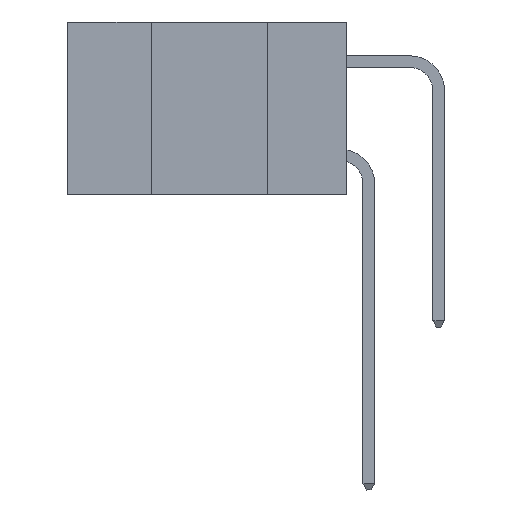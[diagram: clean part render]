
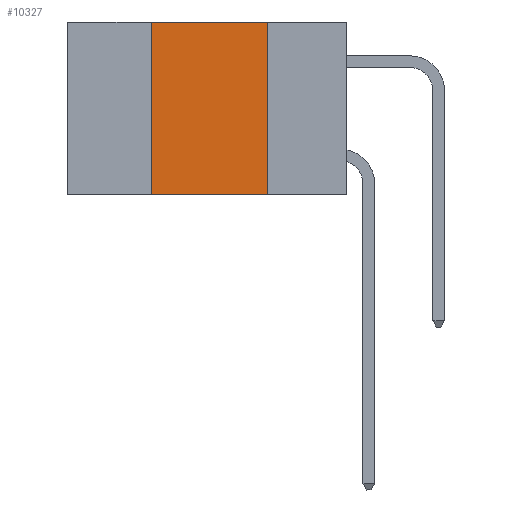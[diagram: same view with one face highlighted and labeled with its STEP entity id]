
A CAD part, left-side view. The second image highlights one B-rep face of the part: STEP entity #10327.
In plain terms, the highlighted planar face has unit normal (-1, 0, 0).
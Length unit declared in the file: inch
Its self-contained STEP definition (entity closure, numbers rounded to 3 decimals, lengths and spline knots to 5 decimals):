
#1672 = CARTESIAN_POINT ( 'NONE',  ( 0., 0.42, -0.37 ) ) ;
#1810 = CARTESIAN_POINT ( 'NONE',  ( 0., 0.42, 0. ) ) ;
#2495 = CARTESIAN_POINT ( 'NONE',  ( 0., 0.6, -0.37 ) ) ;
#2793 = EDGE_CURVE ( 'NONE', #12892, #10421, #13237, .T. ) ;
#3321 = EDGE_CURVE ( 'NONE', #4590, #12892, #12369, .T. ) ;
#3375 = DIRECTION ( 'NONE',  ( 1., 0., 0. ) ) ;
#4590 = VERTEX_POINT ( 'NONE', #1672 ) ;
#4963 = VERTEX_POINT ( 'NONE', #12433 ) ;
#4998 = VECTOR ( 'NONE', #15652, 39.37008 ) ;
#6776 = ORIENTED_EDGE ( 'NONE', *, *, #3321, .F. ) ;
#7063 = ORIENTED_EDGE ( 'NONE', *, *, #2793, .F. ) ;
#7698 = VECTOR ( 'NONE', #20929, 39.37008 ) ;
#10327 = ADVANCED_FACE ( 'NONE', ( #14532 ), #23889, .F. ) ;
#10421 = VERTEX_POINT ( 'NONE', #24111 ) ;
#12037 = LINE ( 'NONE', #20807, #21389 ) ;
#12369 = LINE ( 'NONE', #1810, #21714 ) ;
#12433 = CARTESIAN_POINT ( 'NONE',  ( 0., 0.17, -0.37 ) ) ;
#12531 = EDGE_LOOP ( 'NONE', ( #19228, #7063, #6776, #15261 ) ) ;
#12741 = CARTESIAN_POINT ( 'NONE',  ( 0., 0.42, 0. ) ) ;
#12892 = VERTEX_POINT ( 'NONE', #12741 ) ;
#13075 = DIRECTION ( 'NONE',  ( 0., 0., 1. ) ) ;
#13237 = LINE ( 'NONE', #17187, #7698 ) ;
#14162 = AXIS2_PLACEMENT_3D ( 'NONE', #14653, #3375, #16494 ) ;
#14419 = LINE ( 'NONE', #2495, #4998 ) ;
#14532 = FACE_OUTER_BOUND ( 'NONE', #12531, .T. ) ;
#14653 = CARTESIAN_POINT ( 'NONE',  ( 0., 0.6, 0. ) ) ;
#15261 = ORIENTED_EDGE ( 'NONE', *, *, #21829, .T. ) ;
#15652 = DIRECTION ( 'NONE',  ( 0., -1., 0. ) ) ;
#15908 = EDGE_CURVE ( 'NONE', #10421, #4963, #12037, .T. ) ;
#16494 = DIRECTION ( 'NONE',  ( 0., 0., -1. ) ) ;
#17187 = CARTESIAN_POINT ( 'NONE',  ( 0., 0.6, 0. ) ) ;
#18928 = DIRECTION ( 'NONE',  ( 0., 0., -1. ) ) ;
#19228 = ORIENTED_EDGE ( 'NONE', *, *, #15908, .F. ) ;
#20807 = CARTESIAN_POINT ( 'NONE',  ( 0., 0.17, 0. ) ) ;
#20929 = DIRECTION ( 'NONE',  ( 0., -1., 0. ) ) ;
#21389 = VECTOR ( 'NONE', #18928, 39.37008 ) ;
#21714 = VECTOR ( 'NONE', #13075, 39.37008 ) ;
#21829 = EDGE_CURVE ( 'NONE', #4590, #4963, #14419, .T. ) ;
#23889 = PLANE ( 'NONE',  #14162 ) ;
#24111 = CARTESIAN_POINT ( 'NONE',  ( 0., 0.17, 0. ) ) ;
